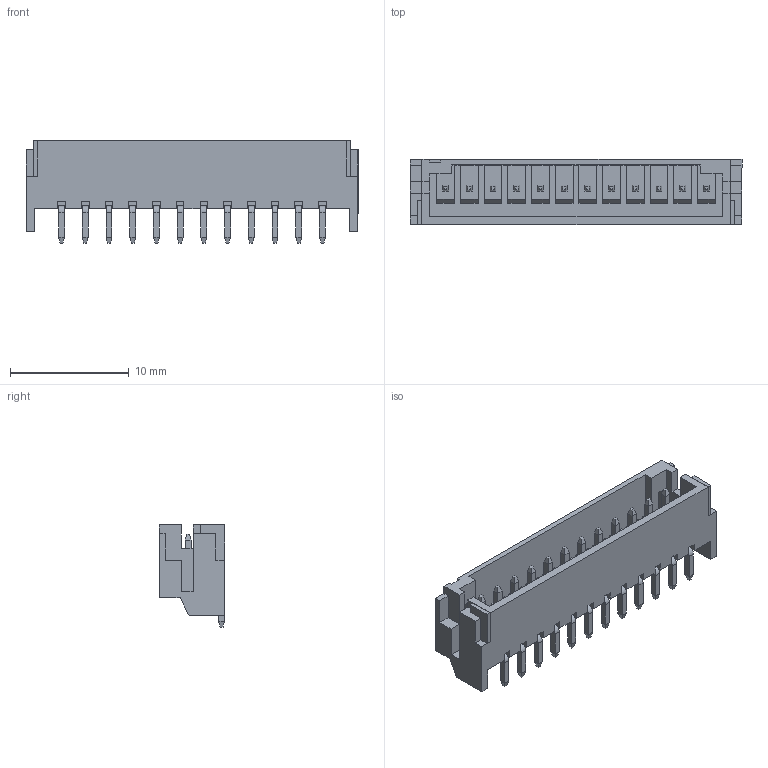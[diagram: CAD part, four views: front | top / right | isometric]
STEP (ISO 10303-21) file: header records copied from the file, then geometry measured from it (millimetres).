
FILE_DESCRIPTION (( 'STEP AP203' ), '1' );
FILE_NAME ('140-512-417-060.STEP', '2020-03-31T20:24:26', ( '' ), ( '' ), 'SwSTEP 2.0', 'SolidWorks 2016', '' );
FILE_SCHEMA (( 'CONFIG_CONTROL_DESIGN' ));
Length unit declared in the file: millimetre
Products named in the file (4): RA SMT Housing_512; 140-512-417-060; RA SMT Pad; RA SMT Contact
Assembly tree (15 placements, depth 2):
  140-512-417-060
    RA SMT Housing_512
    RA SMT Contact  x12
    RA SMT Pad  x2
Bounding box: 28 x 5.5 x 8.65 mm (x, y, z)
Volume: 374.1 mm3; surface area: 1421.5 mm2
Topology: 15 solids, 15 shells, 632 faces, 1528 edges, 922 vertices
Faces by surface type: plane 584, cylinder 48
Entity records: 10354 total; most frequent: CARTESIAN_POINT 1732, ORIENTED_EDGE 1712, DIRECTION 1492, EDGE_CURVE 856, VECTOR 848, LINE 848, VERTEX_POINT 562, AXIS2_PLACEMENT_3D 322
